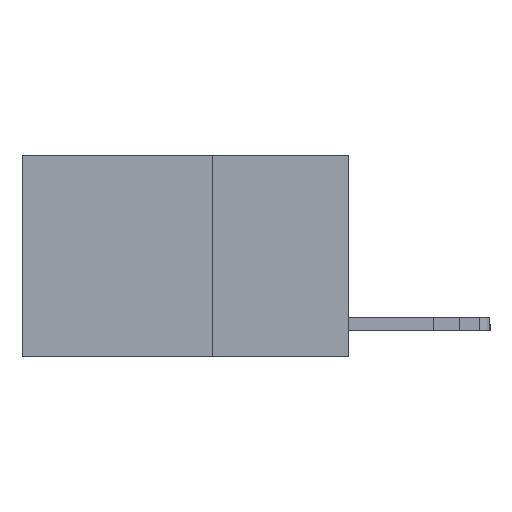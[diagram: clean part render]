
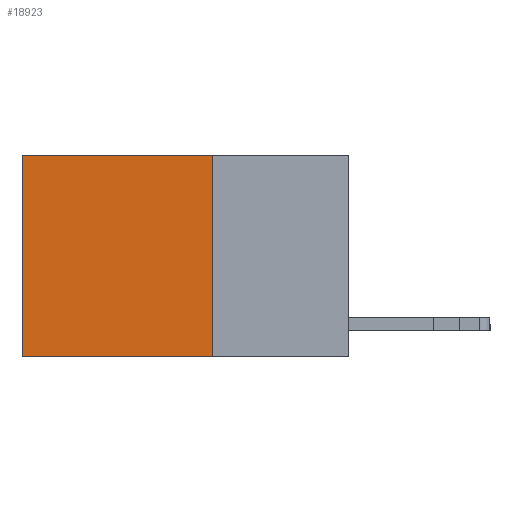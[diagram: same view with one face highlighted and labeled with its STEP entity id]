
A CAD part, left-side view. The second image highlights one B-rep face of the part: STEP entity #18923.
In plain terms, the highlighted planar face has unit normal (-1, 0, 0).
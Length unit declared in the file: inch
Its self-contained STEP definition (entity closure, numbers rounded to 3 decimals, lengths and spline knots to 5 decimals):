
#514 = VERTEX_POINT ( 'NONE', #9690 ) ;
#986 = CARTESIAN_POINT ( 'NONE',  ( 0.2625, 0.25, 0. ) ) ;
#1510 = EDGE_CURVE ( 'NONE', #12771, #514, #8742, .T. ) ;
#3336 = EDGE_CURVE ( 'NONE', #10115, #8892, #3413, .T. ) ;
#3413 = LINE ( 'NONE', #16453, #9137 ) ;
#4730 = VECTOR ( 'NONE', #5546, 39.37008 ) ;
#5082 = ORIENTED_EDGE ( 'NONE', *, *, #6841, .T. ) ;
#5546 = DIRECTION ( 'NONE',  ( 0., 1., 0. ) ) ;
#6841 = EDGE_CURVE ( 'NONE', #514, #8892, #9128, .T. ) ;
#7914 = CARTESIAN_POINT ( 'NONE',  ( 0.2625, 0.6, -0.37 ) ) ;
#8279 = CARTESIAN_POINT ( 'NONE',  ( 0.2625, 0.25, 0. ) ) ;
#8485 = PLANE ( 'NONE',  #14894 ) ;
#8742 = LINE ( 'NONE', #10343, #4730 ) ;
#8751 = ORIENTED_EDGE ( 'NONE', *, *, #3336, .F. ) ;
#8892 = VERTEX_POINT ( 'NONE', #7914 ) ;
#9128 = LINE ( 'NONE', #14162, #14802 ) ;
#9137 = VECTOR ( 'NONE', #13252, 39.37008 ) ;
#9690 = CARTESIAN_POINT ( 'NONE',  ( 0.2625, 0.6, 0. ) ) ;
#10115 = VERTEX_POINT ( 'NONE', #10524 ) ;
#10196 = DIRECTION ( 'NONE',  ( 1., 0., 0. ) ) ;
#10343 = CARTESIAN_POINT ( 'NONE',  ( 0.2625, 0.25, 0. ) ) ;
#10524 = CARTESIAN_POINT ( 'NONE',  ( 0.2625, 0.25, -0.37 ) ) ;
#12771 = VERTEX_POINT ( 'NONE', #986 ) ;
#13252 = DIRECTION ( 'NONE',  ( 0., 1., 0. ) ) ;
#13816 = ORIENTED_EDGE ( 'NONE', *, *, #14480, .F. ) ;
#13822 = EDGE_LOOP ( 'NONE', ( #5082, #8751, #13816, #18279 ) ) ;
#14162 = CARTESIAN_POINT ( 'NONE',  ( 0.2625, 0.6, 0. ) ) ;
#14480 = EDGE_CURVE ( 'NONE', #12771, #10115, #14613, .T. ) ;
#14613 = LINE ( 'NONE', #20919, #19600 ) ;
#14802 = VECTOR ( 'NONE', #15758, 39.37008 ) ;
#14894 = AXIS2_PLACEMENT_3D ( 'NONE', #8279, #10196, #16513 ) ;
#15758 = DIRECTION ( 'NONE',  ( 0., 0., -1. ) ) ;
#16453 = CARTESIAN_POINT ( 'NONE',  ( 0.2625, 0.25, -0.37 ) ) ;
#16513 = DIRECTION ( 'NONE',  ( 0., 0., -1. ) ) ;
#17707 = DIRECTION ( 'NONE',  ( 0., 0., -1. ) ) ;
#18218 = FACE_OUTER_BOUND ( 'NONE', #13822, .T. ) ;
#18279 = ORIENTED_EDGE ( 'NONE', *, *, #1510, .T. ) ;
#18923 = ADVANCED_FACE ( 'NONE', ( #18218 ), #8485, .F. ) ;
#19600 = VECTOR ( 'NONE', #17707, 39.37008 ) ;
#20919 = CARTESIAN_POINT ( 'NONE',  ( 0.2625, 0.25, 0. ) ) ;
